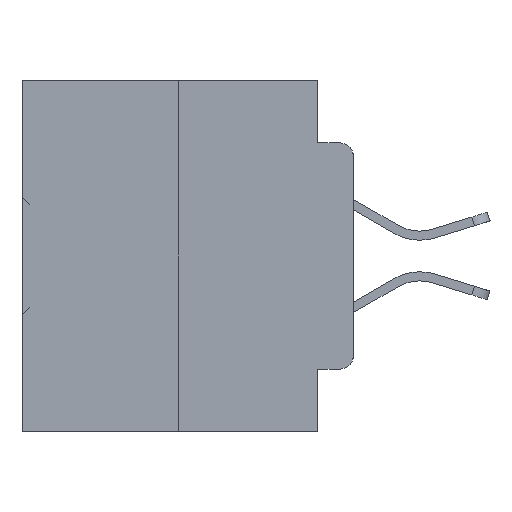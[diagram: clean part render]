
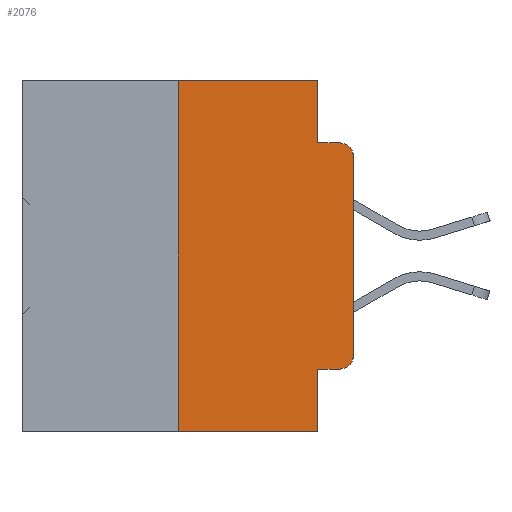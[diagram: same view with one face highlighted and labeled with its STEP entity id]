
A CAD part, left-side view. The second image highlights one B-rep face of the part: STEP entity #2076.
In plain terms, the highlighted planar face has unit normal (-1, 0, 0).
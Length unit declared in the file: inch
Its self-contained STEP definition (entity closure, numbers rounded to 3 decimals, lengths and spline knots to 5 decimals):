
#736 = CARTESIAN_POINT ( 'NONE',  ( 0., 0.25, -0.5 ) ) ;
#2076 = ADVANCED_FACE ( 'NONE', ( #37100 ), #12658, .F. ) ;
#2221 = VECTOR ( 'NONE', #3603, 39.37008 ) ;
#2368 = VERTEX_POINT ( 'NONE', #736 ) ;
#2621 = ORIENTED_EDGE ( 'NONE', *, *, #8544, .T. ) ;
#2724 = EDGE_CURVE ( 'NONE', #2368, #12460, #7966, .T. ) ;
#3119 = ORIENTED_EDGE ( 'NONE', *, *, #2724, .T. ) ;
#3185 = LINE ( 'NONE', #21875, #2221 ) ;
#3603 = DIRECTION ( 'NONE',  ( 0., 0., 1. ) ) ;
#4911 = CARTESIAN_POINT ( 'NONE',  ( 0., 0.02, -0.3915 ) ) ;
#5768 = ORIENTED_EDGE ( 'NONE', *, *, #19552, .F. ) ;
#5930 = CARTESIAN_POINT ( 'NONE',  ( 0., 0.473, -0.5 ) ) ;
#6364 = CARTESIAN_POINT ( 'NONE',  ( 0., 0.051, -0.4115 ) ) ;
#6517 = ORIENTED_EDGE ( 'NONE', *, *, #35875, .F. ) ;
#7236 = EDGE_CURVE ( 'NONE', #20278, #36467, #32455, .T. ) ;
#7426 = VECTOR ( 'NONE', #19276, 39.37008 ) ;
#7935 = DIRECTION ( 'NONE',  ( 0., 0., -1. ) ) ;
#7960 = VERTEX_POINT ( 'NONE', #38501 ) ;
#7963 = VECTOR ( 'NONE', #12629, 39.37008 ) ;
#7966 = LINE ( 'NONE', #5930, #29542 ) ;
#8374 = LINE ( 'NONE', #31487, #22734 ) ;
#8516 = CIRCLE ( 'NONE', #8639, 0.02 ) ;
#8544 = EDGE_CURVE ( 'NONE', #10263, #39262, #8516, .T. ) ;
#8639 = AXIS2_PLACEMENT_3D ( 'NONE', #29413, #11032, #32433 ) ;
#8925 = LINE ( 'NONE', #30947, #7963 ) ;
#8945 = ORIENTED_EDGE ( 'NONE', *, *, #29853, .F. ) ;
#10263 = VERTEX_POINT ( 'NONE', #22013 ) ;
#11032 = DIRECTION ( 'NONE',  ( -1., 0., 0. ) ) ;
#11818 = CARTESIAN_POINT ( 'NONE',  ( 0., 0., -0.3915 ) ) ;
#12460 = VERTEX_POINT ( 'NONE', #26887 ) ;
#12629 = DIRECTION ( 'NONE',  ( 0., 0., 1. ) ) ;
#12658 = PLANE ( 'NONE',  #26007 ) ;
#12913 = EDGE_LOOP ( 'NONE', ( #22812, #2621, #6517, #8945, #21064, #17387, #3119, #5768, #26141, #19177 ) ) ;
#15658 = DIRECTION ( 'NONE',  ( 0., 0., -1. ) ) ;
#15706 = VECTOR ( 'NONE', #21726, 39.37008 ) ;
#16026 = LINE ( 'NONE', #21790, #22241 ) ;
#16588 = LINE ( 'NONE', #20590, #25664 ) ;
#17387 = ORIENTED_EDGE ( 'NONE', *, *, #25692, .F. ) ;
#17493 = EDGE_CURVE ( 'NONE', #21240, #20278, #23806, .T. ) ;
#18790 = EDGE_CURVE ( 'NONE', #36467, #10263, #3185, .T. ) ;
#19177 = ORIENTED_EDGE ( 'NONE', *, *, #7236, .T. ) ;
#19276 = DIRECTION ( 'NONE',  ( 0., 0., -1. ) ) ;
#19489 = CARTESIAN_POINT ( 'NONE',  ( 0., 0.02, -0.4115 ) ) ;
#19552 = EDGE_CURVE ( 'NONE', #21240, #12460, #31856, .T. ) ;
#20278 = VERTEX_POINT ( 'NONE', #19489 ) ;
#20590 = CARTESIAN_POINT ( 'NONE',  ( 0., 0.473, 0. ) ) ;
#21064 = ORIENTED_EDGE ( 'NONE', *, *, #34966, .F. ) ;
#21240 = VERTEX_POINT ( 'NONE', #38343 ) ;
#21726 = DIRECTION ( 'NONE',  ( 0., -1., 0. ) ) ;
#21790 = CARTESIAN_POINT ( 'NONE',  ( 0., 0.051, 0. ) ) ;
#21875 = CARTESIAN_POINT ( 'NONE',  ( 0., 0., 0. ) ) ;
#22013 = CARTESIAN_POINT ( 'NONE',  ( 0., 0., -0.1085 ) ) ;
#22241 = VECTOR ( 'NONE', #15658, 39.37008 ) ;
#22734 = VECTOR ( 'NONE', #34518, 39.37008 ) ;
#22812 = ORIENTED_EDGE ( 'NONE', *, *, #18790, .T. ) ;
#22885 = DIRECTION ( 'NONE',  ( 0., 0., -1. ) ) ;
#22932 = DIRECTION ( 'NONE',  ( 1., 0., 0. ) ) ;
#23806 = LINE ( 'NONE', #6364, #15706 ) ;
#25664 = VECTOR ( 'NONE', #32851, 39.37008 ) ;
#25692 = EDGE_CURVE ( 'NONE', #2368, #35957, #8925, .T. ) ;
#25841 = CARTESIAN_POINT ( 'NONE',  ( 0., 0.25, 0. ) ) ;
#26007 = AXIS2_PLACEMENT_3D ( 'NONE', #35128, #22932, #22885 ) ;
#26141 = ORIENTED_EDGE ( 'NONE', *, *, #17493, .T. ) ;
#26256 = DIRECTION ( 'NONE',  ( -1., 0., 0. ) ) ;
#26887 = CARTESIAN_POINT ( 'NONE',  ( 0., 0.051, -0.5 ) ) ;
#29413 = CARTESIAN_POINT ( 'NONE',  ( 0., 0.02, -0.1085 ) ) ;
#29542 = VECTOR ( 'NONE', #33886, 39.37008 ) ;
#29853 = EDGE_CURVE ( 'NONE', #31501, #7960, #16026, .T. ) ;
#30536 = CARTESIAN_POINT ( 'NONE',  ( 0., 0.051, 0. ) ) ;
#30917 = AXIS2_PLACEMENT_3D ( 'NONE', #4911, #26256, #7935 ) ;
#30947 = CARTESIAN_POINT ( 'NONE',  ( 0., 0.25, 0. ) ) ;
#31487 = CARTESIAN_POINT ( 'NONE',  ( 0., 0.051, -0.0885 ) ) ;
#31501 = VERTEX_POINT ( 'NONE', #30536 ) ;
#31856 = LINE ( 'NONE', #34491, #7426 ) ;
#32433 = DIRECTION ( 'NONE',  ( 0., 0., -1. ) ) ;
#32455 = CIRCLE ( 'NONE', #30917, 0.02 ) ;
#32851 = DIRECTION ( 'NONE',  ( 0., -1., 0. ) ) ;
#33886 = DIRECTION ( 'NONE',  ( 0., -1., 0. ) ) ;
#34491 = CARTESIAN_POINT ( 'NONE',  ( 0., 0.051, 0. ) ) ;
#34518 = DIRECTION ( 'NONE',  ( 0., -1., 0. ) ) ;
#34966 = EDGE_CURVE ( 'NONE', #35957, #31501, #16588, .T. ) ;
#35128 = CARTESIAN_POINT ( 'NONE',  ( 0., 0.473, 0. ) ) ;
#35372 = CARTESIAN_POINT ( 'NONE',  ( 0., 0.02, -0.0885 ) ) ;
#35875 = EDGE_CURVE ( 'NONE', #7960, #39262, #8374, .T. ) ;
#35957 = VERTEX_POINT ( 'NONE', #25841 ) ;
#36467 = VERTEX_POINT ( 'NONE', #11818 ) ;
#37100 = FACE_OUTER_BOUND ( 'NONE', #12913, .T. ) ;
#38343 = CARTESIAN_POINT ( 'NONE',  ( 0., 0.051, -0.4115 ) ) ;
#38501 = CARTESIAN_POINT ( 'NONE',  ( 0., 0.051, -0.0885 ) ) ;
#39262 = VERTEX_POINT ( 'NONE', #35372 ) ;
